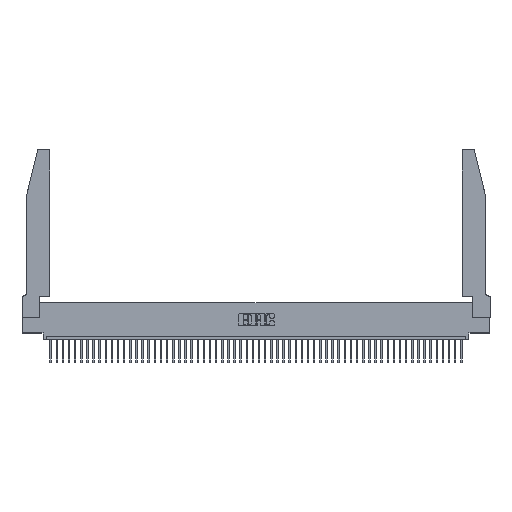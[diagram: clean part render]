
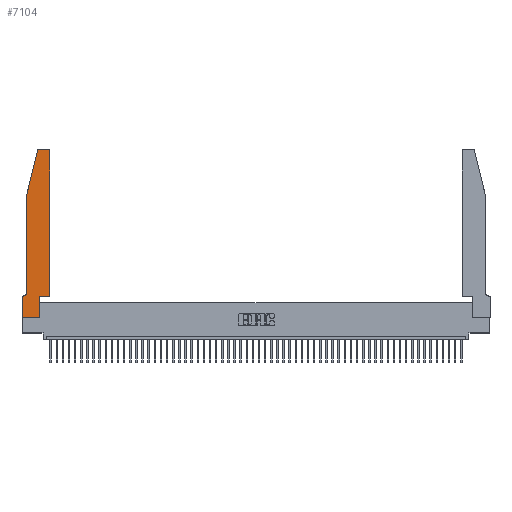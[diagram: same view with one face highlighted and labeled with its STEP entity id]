
A CAD part, top view. The second image highlights one B-rep face of the part: STEP entity #7104.
In plain terms, the highlighted planar face has unit normal (0, 0, 1).
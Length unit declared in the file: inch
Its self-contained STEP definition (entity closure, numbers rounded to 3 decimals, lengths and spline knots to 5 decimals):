
#995 = ORIENTED_EDGE ( 'NONE', *, *, #11313, .T. ) ;
#1000 = ORIENTED_EDGE ( 'NONE', *, *, #43592, .T. ) ;
#1499 = DIRECTION ( 'NONE',  ( -0.239, -0.971, 0. ) ) ;
#1819 = EDGE_CURVE ( 'NONE', #34469, #18894, #34706, .T. ) ;
#2060 = CIRCLE ( 'NONE', #44232, 0.03 ) ;
#2820 = CARTESIAN_POINT ( 'NONE',  ( 0.4505, 2.72, 0.37 ) ) ;
#2972 = EDGE_CURVE ( 'NONE', #18894, #31750, #46787, .T. ) ;
#3785 = CARTESIAN_POINT ( 'NONE',  ( 0.4205, 2.75, 0.37 ) ) ;
#5242 = DIRECTION ( 'NONE',  ( 0., 0., 1. ) ) ;
#7104 = ADVANCED_FACE ( 'NONE', ( #22212 ), #39071, .T. ) ;
#7451 = DIRECTION ( 'NONE',  ( 1., 0., 0. ) ) ;
#7538 = CARTESIAN_POINT ( 'NONE',  ( 0.0055, 0.35, 0.37 ) ) ;
#8008 = VECTOR ( 'NONE', #39461, 39.37008 ) ;
#8137 = CARTESIAN_POINT ( 'NONE',  ( 0.0755, 2., 0.37 ) ) ;
#9088 = ORIENTED_EDGE ( 'NONE', *, *, #2972, .T. ) ;
#9155 = LINE ( 'NONE', #11731, #41018 ) ;
#9204 = CARTESIAN_POINT ( 'NONE',  ( 0.4505, 0.35, 0.37 ) ) ;
#10558 = ORIENTED_EDGE ( 'NONE', *, *, #25069, .T. ) ;
#11313 = EDGE_CURVE ( 'NONE', #14393, #50348, #31960, .T. ) ;
#11658 = ORIENTED_EDGE ( 'NONE', *, *, #1819, .T. ) ;
#11731 = CARTESIAN_POINT ( 'NONE',  ( 0.2605, 2.75, 0.37 ) ) ;
#12228 = ORIENTED_EDGE ( 'NONE', *, *, #13742, .T. ) ;
#12359 = DIRECTION ( 'NONE',  ( 0., 0., -1. ) ) ;
#13742 = EDGE_CURVE ( 'NONE', #31750, #40605, #40020, .T. ) ;
#13889 = EDGE_CURVE ( 'NONE', #51682, #30519, #24703, .T. ) ;
#14036 = VERTEX_POINT ( 'NONE', #46626 ) ;
#14393 = VERTEX_POINT ( 'NONE', #41794 ) ;
#14435 = VECTOR ( 'NONE', #23855, 39.37008 ) ;
#14737 = CARTESIAN_POINT ( 'NONE',  ( 0., 0.35, 0.37 ) ) ;
#15627 = DIRECTION ( 'NONE',  ( 0., 1., 0. ) ) ;
#16101 = DIRECTION ( 'NONE',  ( 1., 0., 0. ) ) ;
#18393 = VECTOR ( 'NONE', #15627, 39.37008 ) ;
#18470 = DIRECTION ( 'NONE',  ( 0., 0., 1. ) ) ;
#18604 = DIRECTION ( 'NONE',  ( 0., -1., 0. ) ) ;
#18894 = VERTEX_POINT ( 'NONE', #19688 ) ;
#19688 = CARTESIAN_POINT ( 'NONE',  ( 0., 0., 0.37 ) ) ;
#20560 = EDGE_CURVE ( 'NONE', #46437, #31971, #9155, .T. ) ;
#20646 = VECTOR ( 'NONE', #40586, 39.37008 ) ;
#21055 = EDGE_CURVE ( 'NONE', #14036, #30808, #37191, .T. ) ;
#21230 = CIRCLE ( 'NONE', #51953, 0.03 ) ;
#21472 = CARTESIAN_POINT ( 'NONE',  ( 0.4205, 2.72, 0.37 ) ) ;
#21637 = CARTESIAN_POINT ( 'NONE',  ( 0.0755, 2., 0.37 ) ) ;
#22212 = FACE_OUTER_BOUND ( 'NONE', #47876, .T. ) ;
#23095 = CARTESIAN_POINT ( 'NONE',  ( 0., 0.35, 0.37 ) ) ;
#23290 = CARTESIAN_POINT ( 'NONE',  ( 0.2865, 0.35, 0.37 ) ) ;
#23855 = DIRECTION ( 'NONE',  ( 1., 0., 0. ) ) ;
#24046 = ORIENTED_EDGE ( 'NONE', *, *, #32760, .T. ) ;
#24152 = CARTESIAN_POINT ( 'NONE',  ( 0., 0., 0.37 ) ) ;
#24703 = LINE ( 'NONE', #9204, #39352 ) ;
#25069 = EDGE_CURVE ( 'NONE', #50348, #14036, #27275, .T. ) ;
#25185 = CARTESIAN_POINT ( 'NONE',  ( 0.0055, 0.42, 0.37 ) ) ;
#25990 = CARTESIAN_POINT ( 'NONE',  ( 0.284, 2.75, 0.37 ) ) ;
#26841 = VECTOR ( 'NONE', #1499, 39.37008 ) ;
#27275 = LINE ( 'NONE', #27702, #38018 ) ;
#27702 = CARTESIAN_POINT ( 'NONE',  ( 0.0755, 2., 0.37 ) ) ;
#30241 = CARTESIAN_POINT ( 'NONE',  ( 0.2865, 0., 0.37 ) ) ;
#30296 = ORIENTED_EDGE ( 'NONE', *, *, #13889, .T. ) ;
#30519 = VERTEX_POINT ( 'NONE', #2820 ) ;
#30808 = VERTEX_POINT ( 'NONE', #7538 ) ;
#31059 = CARTESIAN_POINT ( 'NONE',  ( 0.4505, 0.35, 0.37 ) ) ;
#31750 = VERTEX_POINT ( 'NONE', #30241 ) ;
#31960 = LINE ( 'NONE', #21637, #26841 ) ;
#31971 = VERTEX_POINT ( 'NONE', #25990 ) ;
#32706 = LINE ( 'NONE', #36005, #20646 ) ;
#32760 = EDGE_CURVE ( 'NONE', #30519, #46437, #21230, .T. ) ;
#33372 = DIRECTION ( 'NONE',  ( 0., 1., 0. ) ) ;
#33471 = EDGE_CURVE ( 'NONE', #31971, #14393, #2060, .T. ) ;
#33702 = DIRECTION ( 'NONE',  ( 1., 0., 0. ) ) ;
#34469 = VERTEX_POINT ( 'NONE', #23095 ) ;
#34706 = LINE ( 'NONE', #47746, #8008 ) ;
#35347 = DIRECTION ( 'NONE',  ( 1., 0., 0. ) ) ;
#36005 = CARTESIAN_POINT ( 'NONE',  ( 0.0755, 0.35, 0.37 ) ) ;
#37191 = CIRCLE ( 'NONE', #39325, 0.07 ) ;
#37504 = DIRECTION ( 'NONE',  ( -1., 0., 0. ) ) ;
#38018 = VECTOR ( 'NONE', #18604, 39.37008 ) ;
#38988 = EDGE_CURVE ( 'NONE', #40605, #51682, #47217, .T. ) ;
#39071 = PLANE ( 'NONE',  #48369 ) ;
#39325 = AXIS2_PLACEMENT_3D ( 'NONE', #25185, #12359, #49040 ) ;
#39336 = ORIENTED_EDGE ( 'NONE', *, *, #38988, .T. ) ;
#39352 = VECTOR ( 'NONE', #33372, 39.37008 ) ;
#39461 = DIRECTION ( 'NONE',  ( 0., -1., 0. ) ) ;
#39720 = VECTOR ( 'NONE', #16101, 39.37008 ) ;
#40020 = LINE ( 'NONE', #45725, #18393 ) ;
#40586 = DIRECTION ( 'NONE',  ( -1., 0., 0. ) ) ;
#40605 = VERTEX_POINT ( 'NONE', #23290 ) ;
#41018 = VECTOR ( 'NONE', #37504, 39.37008 ) ;
#41794 = CARTESIAN_POINT ( 'NONE',  ( 0.25487, 2.72718, 0.37 ) ) ;
#43592 = EDGE_CURVE ( 'NONE', #30808, #34469, #32706, .T. ) ;
#43888 = CARTESIAN_POINT ( 'NONE',  ( 0.284, 2.72, 0.37 ) ) ;
#44232 = AXIS2_PLACEMENT_3D ( 'NONE', #43888, #52352, #7451 ) ;
#44911 = ORIENTED_EDGE ( 'NONE', *, *, #21055, .T. ) ;
#45725 = CARTESIAN_POINT ( 'NONE',  ( 0.2865, 0.35, 0.37 ) ) ;
#46437 = VERTEX_POINT ( 'NONE', #3785 ) ;
#46626 = CARTESIAN_POINT ( 'NONE',  ( 0.0755, 0.42, 0.37 ) ) ;
#46787 = LINE ( 'NONE', #24152, #14435 ) ;
#47217 = LINE ( 'NONE', #31059, #39720 ) ;
#47746 = CARTESIAN_POINT ( 'NONE',  ( 0., 0., 0.37 ) ) ;
#47876 = EDGE_LOOP ( 'NONE', ( #51002, #48727, #995, #10558, #44911, #1000, #11658, #9088, #12228, #39336, #30296, #24046 ) ) ;
#48369 = AXIS2_PLACEMENT_3D ( 'NONE', #14737, #18470, #35347 ) ;
#48727 = ORIENTED_EDGE ( 'NONE', *, *, #33471, .T. ) ;
#48732 = CARTESIAN_POINT ( 'NONE',  ( 0.4505, 0.35, 0.37 ) ) ;
#49040 = DIRECTION ( 'NONE',  ( -1., 0., 0. ) ) ;
#50348 = VERTEX_POINT ( 'NONE', #8137 ) ;
#51002 = ORIENTED_EDGE ( 'NONE', *, *, #20560, .T. ) ;
#51682 = VERTEX_POINT ( 'NONE', #48732 ) ;
#51953 = AXIS2_PLACEMENT_3D ( 'NONE', #21472, #5242, #33702 ) ;
#52352 = DIRECTION ( 'NONE',  ( 0., 0., 1. ) ) ;
